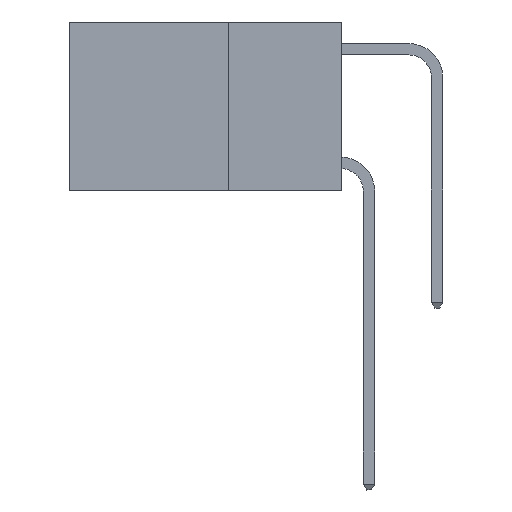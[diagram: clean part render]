
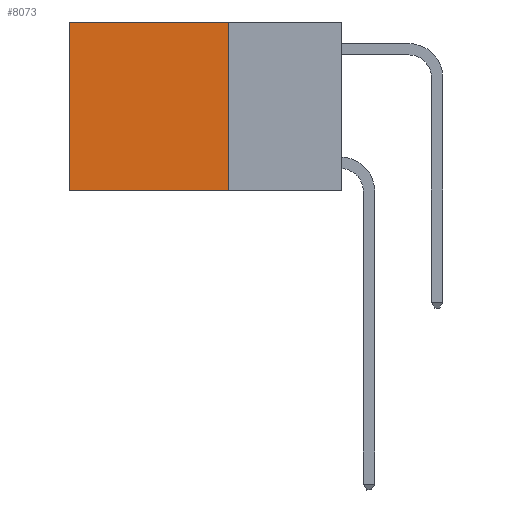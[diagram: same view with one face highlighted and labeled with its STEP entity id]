
A CAD part, left-side view. The second image highlights one B-rep face of the part: STEP entity #8073.
In plain terms, the highlighted planar face has unit normal (-1, 0, 0).
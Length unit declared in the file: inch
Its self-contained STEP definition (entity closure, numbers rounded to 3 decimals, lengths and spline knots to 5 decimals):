
#1600 = CARTESIAN_POINT ( 'NONE',  ( 0.2625, 0.25, 0. ) ) ;
#1717 = VERTEX_POINT ( 'NONE', #14784 ) ;
#2141 = EDGE_LOOP ( 'NONE', ( #19115, #14420, #19714, #15336 ) ) ;
#2246 = DIRECTION ( 'NONE',  ( 0., 0., -1. ) ) ;
#2500 = EDGE_CURVE ( 'NONE', #20313, #7928, #6594, .T. ) ;
#3022 = VERTEX_POINT ( 'NONE', #5971 ) ;
#3604 = CARTESIAN_POINT ( 'NONE',  ( 0.2625, 0.25, 0. ) ) ;
#4815 = DIRECTION ( 'NONE',  ( 0., 1., 0. ) ) ;
#5087 = DIRECTION ( 'NONE',  ( 1., 0., 0. ) ) ;
#5228 = EDGE_CURVE ( 'NONE', #7928, #1717, #5332, .T. ) ;
#5306 = CARTESIAN_POINT ( 'NONE',  ( 0.2625, 0.6, 0. ) ) ;
#5332 = LINE ( 'NONE', #11585, #13934 ) ;
#5971 = CARTESIAN_POINT ( 'NONE',  ( 0.2625, 0.25, -0.37 ) ) ;
#6594 = LINE ( 'NONE', #3604, #8156 ) ;
#7363 = VECTOR ( 'NONE', #15279, 39.37008 ) ;
#7928 = VERTEX_POINT ( 'NONE', #5306 ) ;
#8073 = ADVANCED_FACE ( 'NONE', ( #17540 ), #8172, .F. ) ;
#8156 = VECTOR ( 'NONE', #10253, 39.37008 ) ;
#8172 = PLANE ( 'NONE',  #16374 ) ;
#8627 = EDGE_CURVE ( 'NONE', #3022, #1717, #9424, .T. ) ;
#9424 = LINE ( 'NONE', #15948, #20237 ) ;
#9686 = DIRECTION ( 'NONE',  ( 0., 0., -1. ) ) ;
#10253 = DIRECTION ( 'NONE',  ( 0., 1., 0. ) ) ;
#11585 = CARTESIAN_POINT ( 'NONE',  ( 0.2625, 0.6, 0. ) ) ;
#11975 = LINE ( 'NONE', #19940, #7363 ) ;
#12732 = EDGE_CURVE ( 'NONE', #20313, #3022, #11975, .T. ) ;
#13934 = VECTOR ( 'NONE', #2246, 39.37008 ) ;
#13966 = CARTESIAN_POINT ( 'NONE',  ( 0.2625, 0.25, 0. ) ) ;
#14420 = ORIENTED_EDGE ( 'NONE', *, *, #8627, .F. ) ;
#14784 = CARTESIAN_POINT ( 'NONE',  ( 0.2625, 0.6, -0.37 ) ) ;
#15279 = DIRECTION ( 'NONE',  ( 0., 0., -1. ) ) ;
#15336 = ORIENTED_EDGE ( 'NONE', *, *, #2500, .T. ) ;
#15948 = CARTESIAN_POINT ( 'NONE',  ( 0.2625, 0.25, -0.37 ) ) ;
#16374 = AXIS2_PLACEMENT_3D ( 'NONE', #1600, #5087, #9686 ) ;
#17540 = FACE_OUTER_BOUND ( 'NONE', #2141, .T. ) ;
#19115 = ORIENTED_EDGE ( 'NONE', *, *, #5228, .T. ) ;
#19714 = ORIENTED_EDGE ( 'NONE', *, *, #12732, .F. ) ;
#19940 = CARTESIAN_POINT ( 'NONE',  ( 0.2625, 0.25, 0. ) ) ;
#20237 = VECTOR ( 'NONE', #4815, 39.37008 ) ;
#20313 = VERTEX_POINT ( 'NONE', #13966 ) ;
